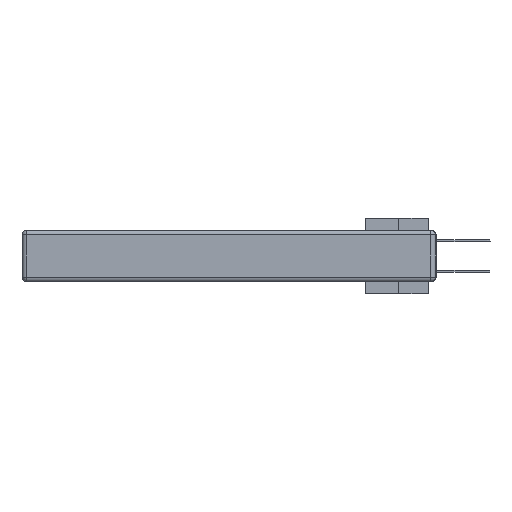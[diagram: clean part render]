
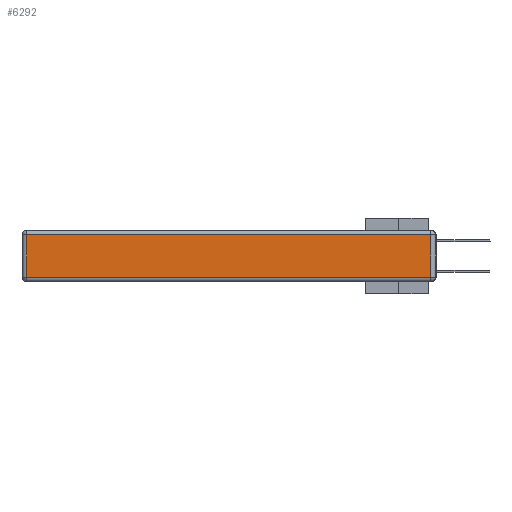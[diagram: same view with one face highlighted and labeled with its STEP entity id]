
A CAD part, left-side view. The second image highlights one B-rep face of the part: STEP entity #6292.
In plain terms, the highlighted planar face has unit normal (-1, 0, 0).
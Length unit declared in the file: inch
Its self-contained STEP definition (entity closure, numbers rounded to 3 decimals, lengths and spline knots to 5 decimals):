
#1732 = CARTESIAN_POINT ( 'NONE',  ( 0., 2.72, -0.313 ) ) ;
#2964 = VERTEX_POINT ( 'NONE', #1732 ) ;
#3468 = VERTEX_POINT ( 'NONE', #30500 ) ;
#3884 = LINE ( 'NONE', #17682, #33063 ) ;
#4171 = EDGE_CURVE ( 'NONE', #2964, #3468, #8358, .T. ) ;
#4889 = AXIS2_PLACEMENT_3D ( 'NONE', #14447, #19703, #7017 ) ;
#5440 = CARTESIAN_POINT ( 'NONE',  ( 0., 0.03, -0.03 ) ) ;
#5618 = ORIENTED_EDGE ( 'NONE', *, *, #9428, .T. ) ;
#6292 = ADVANCED_FACE ( 'NONE', ( #13685 ), #22722, .T. ) ;
#7017 = DIRECTION ( 'NONE',  ( 0., 0., 1. ) ) ;
#7610 = DIRECTION ( 'NONE',  ( 0., 1., 0. ) ) ;
#8358 = LINE ( 'NONE', #27366, #27627 ) ;
#8564 = VECTOR ( 'NONE', #7610, 39.37008 ) ;
#9192 = DIRECTION ( 'NONE',  ( 0., 0., -1. ) ) ;
#9428 = EDGE_CURVE ( 'NONE', #22161, #18381, #27831, .T. ) ;
#11525 = ORIENTED_EDGE ( 'NONE', *, *, #4171, .T. ) ;
#11975 = VECTOR ( 'NONE', #9192, 39.37008 ) ;
#13685 = FACE_OUTER_BOUND ( 'NONE', #29893, .T. ) ;
#14447 = CARTESIAN_POINT ( 'NONE',  ( 0., 0., -0.343 ) ) ;
#14754 = CARTESIAN_POINT ( 'NONE',  ( 0., 2.72, -0.03 ) ) ;
#17682 = CARTESIAN_POINT ( 'NONE',  ( 0., 0.03, -0.343 ) ) ;
#18381 = VERTEX_POINT ( 'NONE', #14754 ) ;
#18925 = LINE ( 'NONE', #30413, #11975 ) ;
#19703 = DIRECTION ( 'NONE',  ( -1., 0., 0. ) ) ;
#20460 = DIRECTION ( 'NONE',  ( 0., 0., 1. ) ) ;
#21844 = ORIENTED_EDGE ( 'NONE', *, *, #25669, .T. ) ;
#22161 = VERTEX_POINT ( 'NONE', #5440 ) ;
#22722 = PLANE ( 'NONE',  #4889 ) ;
#23202 = CARTESIAN_POINT ( 'NONE',  ( 0., 2.75, -0.03 ) ) ;
#23980 = EDGE_CURVE ( 'NONE', #3468, #22161, #3884, .T. ) ;
#24254 = ORIENTED_EDGE ( 'NONE', *, *, #23980, .T. ) ;
#24614 = DIRECTION ( 'NONE',  ( 0., -1., 0. ) ) ;
#25669 = EDGE_CURVE ( 'NONE', #18381, #2964, #18925, .T. ) ;
#27366 = CARTESIAN_POINT ( 'NONE',  ( 0., 0., -0.313 ) ) ;
#27627 = VECTOR ( 'NONE', #24614, 39.37008 ) ;
#27831 = LINE ( 'NONE', #23202, #8564 ) ;
#29893 = EDGE_LOOP ( 'NONE', ( #11525, #24254, #5618, #21844 ) ) ;
#30413 = CARTESIAN_POINT ( 'NONE',  ( 0., 2.72, -0.343 ) ) ;
#30500 = CARTESIAN_POINT ( 'NONE',  ( 0., 0.03, -0.313 ) ) ;
#33063 = VECTOR ( 'NONE', #20460, 39.37008 ) ;
